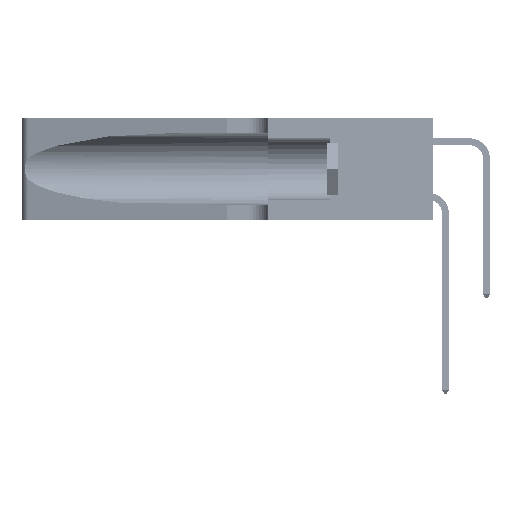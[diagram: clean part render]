
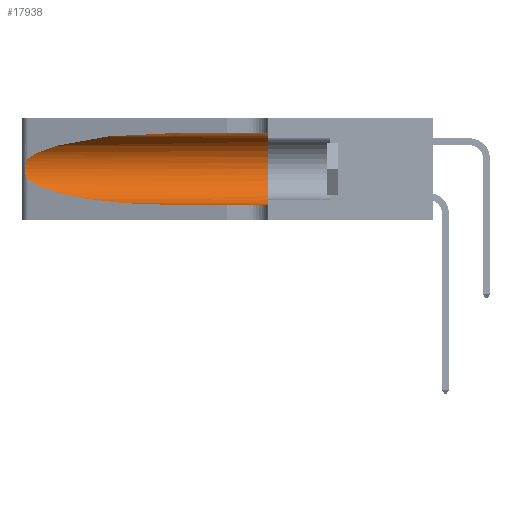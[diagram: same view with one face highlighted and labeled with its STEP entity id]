
A CAD part, left-side view. The second image highlights one B-rep face of the part: STEP entity #17938.
In plain terms, the highlighted cylindrical face has radius 3.308 mm (diameter 6.617 mm), a partial arc.
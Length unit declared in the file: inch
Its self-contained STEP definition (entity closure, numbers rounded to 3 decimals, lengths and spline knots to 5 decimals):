
#260 = EDGE_CURVE ( 'NONE', #14030, #46147, #4564, .T. ) ;
#1149 = DIRECTION ( 'NONE',  ( 0., 0., 1. ) ) ;
#2080 = CARTESIAN_POINT ( 'NONE',  ( 0.2373, 1.15595, 0.28018 ) ) ;
#2118 = CARTESIAN_POINT ( 'NONE',  ( 0.1305, 1.61858, 0.05475 ) ) ;
#4564 = B_SPLINE_CURVE_WITH_KNOTS ( 'NONE', 3,
 ( #51472, #51639, #31255, #6699, #35375, #10822, #39465, #14960, #43561, #19086, #47693, #23215, #51821, #27355 ),
 .UNSPECIFIED., .F., .F.,
 ( 4, 2, 2, 2, 2, 2, 4 ),
 ( 0., 0.00027, 0.00053, 0.00107, 0.0016, 0.00187, 0.00214 ),
 .UNSPECIFIED. ) ;
#5001 = EDGE_CURVE ( 'NONE', #43379, #6928, #19347, .T. ) ;
#5300 = CARTESIAN_POINT ( 'NONE',  ( 0.2373, 1.15595, 0.08982 ) ) ;
#5657 = ORIENTED_EDGE ( 'NONE', *, *, #260, .T. ) ;
#6699 = CARTESIAN_POINT ( 'NONE',  ( 0.25787, 1.23484, 0.2124 ) ) ;
#6928 = VERTEX_POINT ( 'NONE', #22903 ) ;
#7124 = CIRCLE ( 'NONE', #24745, 0.13025 ) ;
#7285 = VERTEX_POINT ( 'NONE', #8716 ) ;
#7666 = DIRECTION ( 'NONE',  ( 0., -1., 0. ) ) ;
#7878 = VECTOR ( 'NONE', #51379, 39.37008 ) ;
#8716 = CARTESIAN_POINT ( 'NONE',  ( 0.1305, 0.35, 0.05475 ) ) ;
#10822 = CARTESIAN_POINT ( 'NONE',  ( 0.26018, 1.23835, 0.19895 ) ) ;
#13483 = CARTESIAN_POINT ( 'NONE',  ( 0.1305, 0.72297, 0.05475 ) ) ;
#13522 = CARTESIAN_POINT ( 'NONE',  ( 0.18966, 0.96281, 0.05475 ) ) ;
#13535 = EDGE_CURVE ( 'NONE', #6928, #7285, #7124, .T. ) ;
#14030 = VERTEX_POINT ( 'NONE', #36948 ) ;
#14287 = CARTESIAN_POINT ( 'NONE',  ( 0.18966, 0.96281, 0.31525 ) ) ;
#14960 = CARTESIAN_POINT ( 'NONE',  ( 0.26075, 1.23896, 0.178 ) ) ;
#15718 =( BOUNDED_CURVE ( )  B_SPLINE_CURVE ( 3, ( #33948, #5300, #13522, #42133 ),
 .UNSPECIFIED., .F., .F. ) 
 B_SPLINE_CURVE_WITH_KNOTS ( ( 4, 4 ),
 ( 3.44316, 4.71239 ),
 .UNSPECIFIED. ) 
 CURVE ( )  GEOMETRIC_REPRESENTATION_ITEM ( )  RATIONAL_B_SPLINE_CURVE ( ( 1., 0.87, 0.87, 1. ) ) 
 REPRESENTATION_ITEM ( '' )  );
#16738 = ORIENTED_EDGE ( 'NONE', *, *, #22192, .T. ) ;
#17938 = ADVANCED_FACE ( 'NONE', ( #50918 ), #37474, .F. ) ;
#18419 = CARTESIAN_POINT ( 'NONE',  ( 0.1305, 0.72297, 0.31525 ) ) ;
#19086 = CARTESIAN_POINT ( 'NONE',  ( 0.25856, 1.23593, 0.16098 ) ) ;
#19347 = LINE ( 'NONE', #28055, #39807 ) ;
#20827 = ORIENTED_EDGE ( 'NONE', *, *, #23614, .T. ) ;
#22192 = EDGE_CURVE ( 'NONE', #43379, #14030, #25281, .T. ) ;
#22903 = CARTESIAN_POINT ( 'NONE',  ( 0.1305, 0.35, 0.31525 ) ) ;
#23215 = CARTESIAN_POINT ( 'NONE',  ( 0.25639, 1.23186, 0.15144 ) ) ;
#23465 = AXIS2_PLACEMENT_3D ( 'NONE', #52607, #7666, #32216 ) ;
#23614 = EDGE_CURVE ( 'NONE', #46147, #24195, #15718, .T. ) ;
#23716 = CARTESIAN_POINT ( 'NONE',  ( 0.1305, 0.72297, 0.31525 ) ) ;
#24195 = VERTEX_POINT ( 'NONE', #13483 ) ;
#24745 = AXIS2_PLACEMENT_3D ( 'NONE', #50238, #25759, #1149 ) ;
#25281 =( BOUNDED_CURVE ( )  B_SPLINE_CURVE ( 3, ( #18419, #14287, #2080, #30769 ),
 .UNSPECIFIED., .F., .T. ) 
 B_SPLINE_CURVE_WITH_KNOTS ( ( 4, 4 ),
 ( 1.5708, 2.84003 ),
 .UNSPECIFIED. ) 
 CURVE ( )  GEOMETRIC_REPRESENTATION_ITEM ( )  RATIONAL_B_SPLINE_CURVE ( ( 1., 0.87, 0.87, 1. ) ) 
 REPRESENTATION_ITEM ( '' )  );
#25759 = DIRECTION ( 'NONE',  ( 0., 1., 0. ) ) ;
#27020 = ORIENTED_EDGE ( 'NONE', *, *, #5001, .F. ) ;
#27355 = CARTESIAN_POINT ( 'NONE',  ( 0.25487, 1.22718, 0.14631 ) ) ;
#27527 = EDGE_CURVE ( 'NONE', #24195, #7285, #29670, .T. ) ;
#28055 = CARTESIAN_POINT ( 'NONE',  ( 0.1305, 1.61858, 0.31525 ) ) ;
#29670 = LINE ( 'NONE', #2118, #7878 ) ;
#30769 = CARTESIAN_POINT ( 'NONE',  ( 0.25487, 1.22718, 0.22369 ) ) ;
#31255 = CARTESIAN_POINT ( 'NONE',  ( 0.25639, 1.23184, 0.21858 ) ) ;
#32216 = DIRECTION ( 'NONE',  ( 0., 0., -1. ) ) ;
#33948 = CARTESIAN_POINT ( 'NONE',  ( 0.25487, 1.22718, 0.14631 ) ) ;
#35375 = CARTESIAN_POINT ( 'NONE',  ( 0.25854, 1.2359, 0.20912 ) ) ;
#36948 = CARTESIAN_POINT ( 'NONE',  ( 0.25487, 1.22718, 0.22369 ) ) ;
#37474 = CYLINDRICAL_SURFACE ( 'NONE', #23465, 0.13025 ) ;
#37526 = ORIENTED_EDGE ( 'NONE', *, *, #27527, .T. ) ;
#39465 = CARTESIAN_POINT ( 'NONE',  ( 0.26075, 1.23896, 0.19203 ) ) ;
#39807 = VECTOR ( 'NONE', #40355, 39.37008 ) ;
#40355 = DIRECTION ( 'NONE',  ( 0., -1., 0. ) ) ;
#42133 = CARTESIAN_POINT ( 'NONE',  ( 0.1305, 0.72297, 0.05475 ) ) ;
#43379 = VERTEX_POINT ( 'NONE', #23716 ) ;
#43561 = CARTESIAN_POINT ( 'NONE',  ( 0.26017, 1.23833, 0.17102 ) ) ;
#44319 = ORIENTED_EDGE ( 'NONE', *, *, #13535, .F. ) ;
#44553 = EDGE_LOOP ( 'NONE', ( #16738, #5657, #20827, #37526, #44319, #27020 ) ) ;
#46147 = VERTEX_POINT ( 'NONE', #47405 ) ;
#47405 = CARTESIAN_POINT ( 'NONE',  ( 0.25487, 1.22718, 0.14631 ) ) ;
#47693 = CARTESIAN_POINT ( 'NONE',  ( 0.25789, 1.23486, 0.15765 ) ) ;
#50238 = CARTESIAN_POINT ( 'NONE',  ( 0.1305, 0.35, 0.185 ) ) ;
#50918 = FACE_OUTER_BOUND ( 'NONE', #44553, .T. ) ;
#51379 = DIRECTION ( 'NONE',  ( 0., -1., 0. ) ) ;
#51472 = CARTESIAN_POINT ( 'NONE',  ( 0.25487, 1.22718, 0.22369 ) ) ;
#51639 = CARTESIAN_POINT ( 'NONE',  ( 0.25555, 1.22994, 0.2215 ) ) ;
#51821 = CARTESIAN_POINT ( 'NONE',  ( 0.25555, 1.22993, 0.14849 ) ) ;
#52607 = CARTESIAN_POINT ( 'NONE',  ( 0.1305, 1.61858, 0.185 ) ) ;
